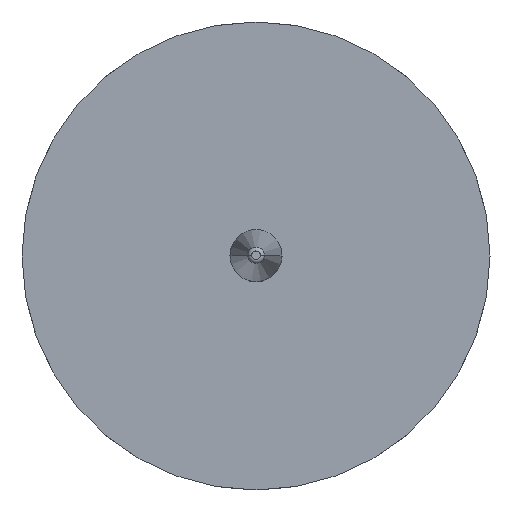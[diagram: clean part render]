
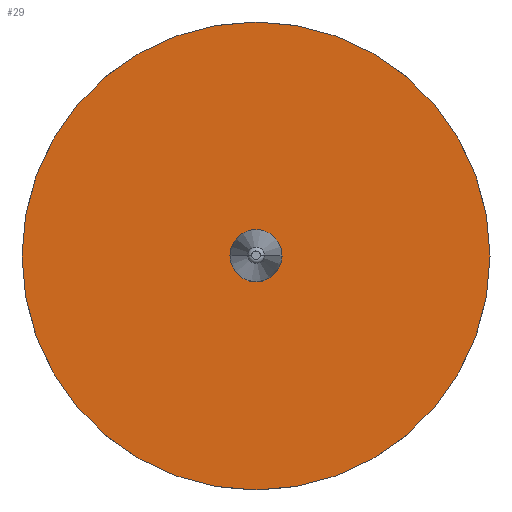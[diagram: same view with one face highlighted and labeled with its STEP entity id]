
A CAD part, top view. The second image highlights one B-rep face of the part: STEP entity #29.
In plain terms, the highlighted planar face has unit normal (0, 0, 1).
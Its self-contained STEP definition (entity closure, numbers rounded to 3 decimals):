
#7 = VERTEX_POINT ( 'NONE', #153 ) ;
#11 = PLANE ( 'NONE',  #295 ) ;
#29 = ADVANCED_FACE ( 'NONE', ( #223, #582 ), #11, .F. ) ;
#59 = ORIENTED_EDGE ( 'NONE', *, *, #346, .T. ) ;
#67 = EDGE_CURVE ( 'NONE', #7, #317, #100, .T. ) ;
#83 = AXIS2_PLACEMENT_3D ( 'NONE', #415, #137, #462 ) ;
#100 = CIRCLE ( 'NONE', #327, 0.5 ) ;
#106 = DIRECTION ( 'NONE',  ( 0., 0., -1. ) ) ;
#108 = DIRECTION ( 'NONE',  ( 0., 0., 1. ) ) ;
#137 = DIRECTION ( 'NONE',  ( 0., 0., 1. ) ) ;
#143 = AXIS2_PLACEMENT_3D ( 'NONE', #465, #178, #517 ) ;
#153 = CARTESIAN_POINT ( 'NONE',  ( -0.5, 0., 0. ) ) ;
#165 = ORIENTED_EDGE ( 'NONE', *, *, #569, .T. ) ;
#169 = CARTESIAN_POINT ( 'NONE',  ( 4.5, 0., 0. ) ) ;
#178 = DIRECTION ( 'NONE',  ( 0., 0., 1. ) ) ;
#179 = VERTEX_POINT ( 'NONE', #169 ) ;
#194 = CIRCLE ( 'NONE', #83, 0.5 ) ;
#223 = FACE_BOUND ( 'NONE', #575, .T. ) ;
#224 = CIRCLE ( 'NONE', #347, 4.5 ) ;
#225 = ORIENTED_EDGE ( 'NONE', *, *, #67, .F. ) ;
#260 = DIRECTION ( 'NONE',  ( 0., 0., 1. ) ) ;
#269 = CIRCLE ( 'NONE', #143, 4.5 ) ;
#281 = EDGE_CURVE ( 'NONE', #317, #7, #194, .T. ) ;
#287 = CARTESIAN_POINT ( 'NONE',  ( 0., 0., 0. ) ) ;
#290 = ORIENTED_EDGE ( 'NONE', *, *, #281, .F. ) ;
#295 = AXIS2_PLACEMENT_3D ( 'NONE', #287, #106, #430 ) ;
#317 = VERTEX_POINT ( 'NONE', #366 ) ;
#327 = AXIS2_PLACEMENT_3D ( 'NONE', #492, #260, #495 ) ;
#346 = EDGE_CURVE ( 'NONE', #525, #179, #269, .T. ) ;
#347 = AXIS2_PLACEMENT_3D ( 'NONE', #388, #108, #435 ) ;
#366 = CARTESIAN_POINT ( 'NONE',  ( 0.5, 0., 0. ) ) ;
#388 = CARTESIAN_POINT ( 'NONE',  ( 0., 0., 0. ) ) ;
#415 = CARTESIAN_POINT ( 'NONE',  ( 0., 0., 0. ) ) ;
#430 = DIRECTION ( 'NONE',  ( -1., 0., 0. ) ) ;
#435 = DIRECTION ( 'NONE',  ( 1., 0., 0. ) ) ;
#462 = DIRECTION ( 'NONE',  ( 1., 0., 0. ) ) ;
#465 = CARTESIAN_POINT ( 'NONE',  ( 0., 0., 0. ) ) ;
#479 = CARTESIAN_POINT ( 'NONE',  ( -4.5, 0., 0. ) ) ;
#492 = CARTESIAN_POINT ( 'NONE',  ( 0., 0., 0. ) ) ;
#495 = DIRECTION ( 'NONE',  ( 1., 0., 0. ) ) ;
#517 = DIRECTION ( 'NONE',  ( 1., 0., 0. ) ) ;
#525 = VERTEX_POINT ( 'NONE', #479 ) ;
#552 = EDGE_LOOP ( 'NONE', ( #165, #59 ) ) ;
#569 = EDGE_CURVE ( 'NONE', #179, #525, #224, .T. ) ;
#575 = EDGE_LOOP ( 'NONE', ( #290, #225 ) ) ;
#582 = FACE_OUTER_BOUND ( 'NONE', #552, .T. ) ;
